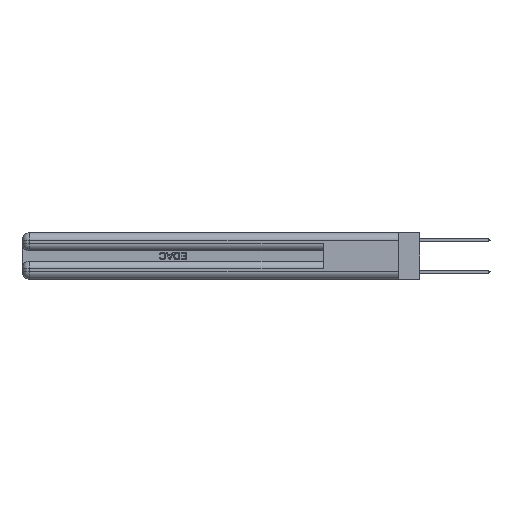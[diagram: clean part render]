
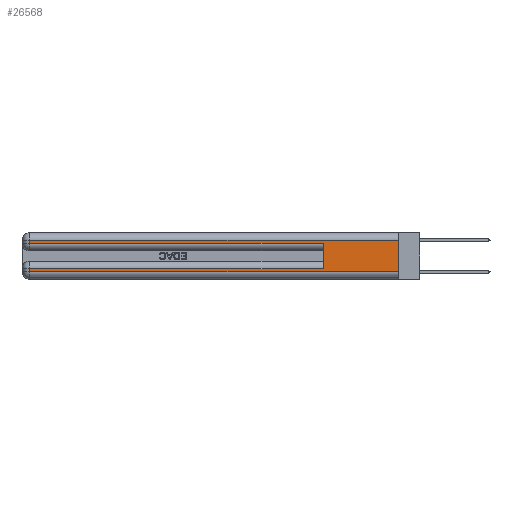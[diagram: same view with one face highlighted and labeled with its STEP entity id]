
A CAD part, left-side view. The second image highlights one B-rep face of the part: STEP entity #26568.
In plain terms, the highlighted planar face has unit normal (-1, 0, 0).
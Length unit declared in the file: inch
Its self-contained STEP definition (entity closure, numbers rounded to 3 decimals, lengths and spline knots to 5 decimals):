
#579 = CARTESIAN_POINT ( 'NONE',  ( 0., 0., 0.285 ) ) ;
#812 = LINE ( 'NONE', #27568, #943 ) ;
#933 = LINE ( 'NONE', #579, #17906 ) ;
#943 = VECTOR ( 'NONE', #5749, 39.37008 ) ;
#1006 = VECTOR ( 'NONE', #18916, 39.37008 ) ;
#1226 = CARTESIAN_POINT ( 'NONE',  ( 0., 0., 0.37 ) ) ;
#1290 = EDGE_CURVE ( 'NONE', #8004, #8363, #29284, .T. ) ;
#1575 = VERTEX_POINT ( 'NONE', #3396 ) ;
#3124 = VERTEX_POINT ( 'NONE', #15297 ) ;
#3396 = CARTESIAN_POINT ( 'NONE',  ( 0., 0.6, 0.285 ) ) ;
#3524 = DIRECTION ( 'NONE',  ( 1., 0., 0. ) ) ;
#3870 = PLANE ( 'NONE',  #7827 ) ;
#4624 = ORIENTED_EDGE ( 'NONE', *, *, #17816, .T. ) ;
#5521 = DIRECTION ( 'NONE',  ( 0., -1., 0. ) ) ;
#5623 = CARTESIAN_POINT ( 'NONE',  ( 0., 2.94, 0.37 ) ) ;
#5749 = DIRECTION ( 'NONE',  ( 0., 1., 0. ) ) ;
#6581 = VERTEX_POINT ( 'NONE', #23145 ) ;
#6964 = LINE ( 'NONE', #23333, #28911 ) ;
#7377 = EDGE_CURVE ( 'NONE', #8004, #3124, #12987, .T. ) ;
#7827 = AXIS2_PLACEMENT_3D ( 'NONE', #1226, #3524, #14608 ) ;
#8004 = VERTEX_POINT ( 'NONE', #14668 ) ;
#8236 = VECTOR ( 'NONE', #10982, 39.37008 ) ;
#8363 = VERTEX_POINT ( 'NONE', #15890 ) ;
#10140 = CARTESIAN_POINT ( 'NONE',  ( 0., 0.6, 0.085 ) ) ;
#10459 = LINE ( 'NONE', #12930, #8236 ) ;
#10636 = DIRECTION ( 'NONE',  ( 0., 0., -1. ) ) ;
#10982 = DIRECTION ( 'NONE',  ( 0., 0., -1. ) ) ;
#11154 = LINE ( 'NONE', #11509, #1006 ) ;
#11301 = VECTOR ( 'NONE', #20910, 39.37008 ) ;
#11509 = CARTESIAN_POINT ( 'NONE',  ( 0., 0., 0.06 ) ) ;
#11800 = FACE_OUTER_BOUND ( 'NONE', #19617, .T. ) ;
#12032 = EDGE_CURVE ( 'NONE', #25914, #8363, #11154, .T. ) ;
#12278 = CARTESIAN_POINT ( 'NONE',  ( 0., 0., 0.37 ) ) ;
#12812 = CARTESIAN_POINT ( 'NONE',  ( 0., 0., 0.31 ) ) ;
#12930 = CARTESIAN_POINT ( 'NONE',  ( 0., 2.94, 0.37 ) ) ;
#12987 = LINE ( 'NONE', #12812, #11301 ) ;
#13384 = EDGE_CURVE ( 'NONE', #6581, #1575, #933, .T. ) ;
#14141 = CARTESIAN_POINT ( 'NONE',  ( 0., 2.94, 0.085 ) ) ;
#14608 = DIRECTION ( 'NONE',  ( 0., 0., -1. ) ) ;
#14668 = CARTESIAN_POINT ( 'NONE',  ( 0., 0., 0.31 ) ) ;
#15297 = CARTESIAN_POINT ( 'NONE',  ( 0., 2.94, 0.31 ) ) ;
#15603 = ORIENTED_EDGE ( 'NONE', *, *, #7377, .T. ) ;
#15890 = CARTESIAN_POINT ( 'NONE',  ( 0., 0., 0.06 ) ) ;
#16374 = DIRECTION ( 'NONE',  ( 0., 0., -1. ) ) ;
#17139 = EDGE_CURVE ( 'NONE', #26708, #1575, #6964, .T. ) ;
#17364 = DIRECTION ( 'NONE',  ( 0., 0., 1. ) ) ;
#17816 = EDGE_CURVE ( 'NONE', #19430, #25914, #32004, .T. ) ;
#17858 = ORIENTED_EDGE ( 'NONE', *, *, #21974, .T. ) ;
#17906 = VECTOR ( 'NONE', #5521, 39.37008 ) ;
#18916 = DIRECTION ( 'NONE',  ( 0., -1., 0. ) ) ;
#19327 = EDGE_CURVE ( 'NONE', #3124, #6581, #10459, .T. ) ;
#19430 = VERTEX_POINT ( 'NONE', #14141 ) ;
#19617 = EDGE_LOOP ( 'NONE', ( #28071, #15603, #28837, #34609, #23578, #17858, #4624, #29943 ) ) ;
#20910 = DIRECTION ( 'NONE',  ( 0., 1., 0. ) ) ;
#21974 = EDGE_CURVE ( 'NONE', #26708, #19430, #812, .T. ) ;
#23145 = CARTESIAN_POINT ( 'NONE',  ( 0., 2.94, 0.285 ) ) ;
#23333 = CARTESIAN_POINT ( 'NONE',  ( 0., 0.6, 0.145 ) ) ;
#23578 = ORIENTED_EDGE ( 'NONE', *, *, #17139, .F. ) ;
#24277 = VECTOR ( 'NONE', #10636, 39.37008 ) ;
#25577 = VECTOR ( 'NONE', #16374, 39.37008 ) ;
#25914 = VERTEX_POINT ( 'NONE', #27329 ) ;
#26568 = ADVANCED_FACE ( 'NONE', ( #11800 ), #3870, .F. ) ;
#26708 = VERTEX_POINT ( 'NONE', #10140 ) ;
#27329 = CARTESIAN_POINT ( 'NONE',  ( 0., 2.94, 0.06 ) ) ;
#27568 = CARTESIAN_POINT ( 'NONE',  ( 0., 0., 0.085 ) ) ;
#28071 = ORIENTED_EDGE ( 'NONE', *, *, #1290, .F. ) ;
#28837 = ORIENTED_EDGE ( 'NONE', *, *, #19327, .T. ) ;
#28911 = VECTOR ( 'NONE', #17364, 39.37008 ) ;
#29284 = LINE ( 'NONE', #12278, #24277 ) ;
#29943 = ORIENTED_EDGE ( 'NONE', *, *, #12032, .T. ) ;
#32004 = LINE ( 'NONE', #5623, #25577 ) ;
#34609 = ORIENTED_EDGE ( 'NONE', *, *, #13384, .T. ) ;
